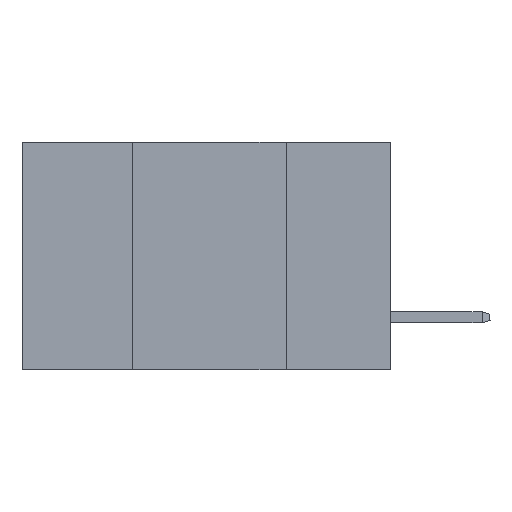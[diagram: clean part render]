
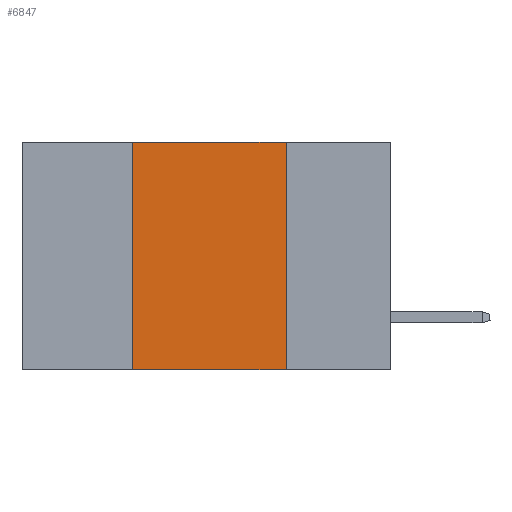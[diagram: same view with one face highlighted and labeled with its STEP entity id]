
A CAD part, left-side view. The second image highlights one B-rep face of the part: STEP entity #6847.
In plain terms, the highlighted planar face has unit normal (-1, 0, 0).
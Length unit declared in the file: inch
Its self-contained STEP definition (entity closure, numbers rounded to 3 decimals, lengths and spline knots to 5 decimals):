
#388 = VERTEX_POINT ( 'NONE', #32428 ) ;
#610 = LINE ( 'NONE', #13097, #8810 ) ;
#3631 = DIRECTION ( 'NONE',  ( 0., 0., 1. ) ) ;
#3962 = VECTOR ( 'NONE', #17994, 39.37008 ) ;
#4367 = ORIENTED_EDGE ( 'NONE', *, *, #20839, .F. ) ;
#4401 = VERTEX_POINT ( 'NONE', #41159 ) ;
#6047 = LINE ( 'NONE', #22054, #23561 ) ;
#6847 = ADVANCED_FACE ( 'NONE', ( #32868 ), #18361, .F. ) ;
#8704 = LINE ( 'NONE', #12960, #11736 ) ;
#8810 = VECTOR ( 'NONE', #3631, 39.37008 ) ;
#9434 = VERTEX_POINT ( 'NONE', #36036 ) ;
#10117 = DIRECTION ( 'NONE',  ( 0., -1., 0. ) ) ;
#10139 = VERTEX_POINT ( 'NONE', #11839 ) ;
#11704 = EDGE_CURVE ( 'NONE', #4401, #9434, #610, .T. ) ;
#11736 = VECTOR ( 'NONE', #10117, 39.37008 ) ;
#11839 = CARTESIAN_POINT ( 'NONE',  ( 0., 0.17, -0.37 ) ) ;
#12960 = CARTESIAN_POINT ( 'NONE',  ( 0., 0.6, -0.37 ) ) ;
#13097 = CARTESIAN_POINT ( 'NONE',  ( 0., 0.42, 0. ) ) ;
#14820 = DIRECTION ( 'NONE',  ( 1., 0., 0. ) ) ;
#16101 = LINE ( 'NONE', #16551, #3962 ) ;
#16551 = CARTESIAN_POINT ( 'NONE',  ( 0., 0.6, 0. ) ) ;
#17987 = AXIS2_PLACEMENT_3D ( 'NONE', #27627, #14820, #18076 ) ;
#17994 = DIRECTION ( 'NONE',  ( 0., -1., 0. ) ) ;
#18076 = DIRECTION ( 'NONE',  ( 0., 0., -1. ) ) ;
#18361 = PLANE ( 'NONE',  #17987 ) ;
#20839 = EDGE_CURVE ( 'NONE', #9434, #388, #16101, .T. ) ;
#22054 = CARTESIAN_POINT ( 'NONE',  ( 0., 0.17, 0. ) ) ;
#23561 = VECTOR ( 'NONE', #35295, 39.37008 ) ;
#26745 = ORIENTED_EDGE ( 'NONE', *, *, #40154, .F. ) ;
#27627 = CARTESIAN_POINT ( 'NONE',  ( 0., 0.6, 0. ) ) ;
#32428 = CARTESIAN_POINT ( 'NONE',  ( 0., 0.17, 0. ) ) ;
#32868 = FACE_OUTER_BOUND ( 'NONE', #40906, .T. ) ;
#33863 = EDGE_CURVE ( 'NONE', #4401, #10139, #8704, .T. ) ;
#35295 = DIRECTION ( 'NONE',  ( 0., 0., -1. ) ) ;
#36036 = CARTESIAN_POINT ( 'NONE',  ( 0., 0.42, 0. ) ) ;
#38001 = ORIENTED_EDGE ( 'NONE', *, *, #11704, .F. ) ;
#39463 = ORIENTED_EDGE ( 'NONE', *, *, #33863, .T. ) ;
#40154 = EDGE_CURVE ( 'NONE', #388, #10139, #6047, .T. ) ;
#40906 = EDGE_LOOP ( 'NONE', ( #26745, #4367, #38001, #39463 ) ) ;
#41159 = CARTESIAN_POINT ( 'NONE',  ( 0., 0.42, -0.37 ) ) ;
